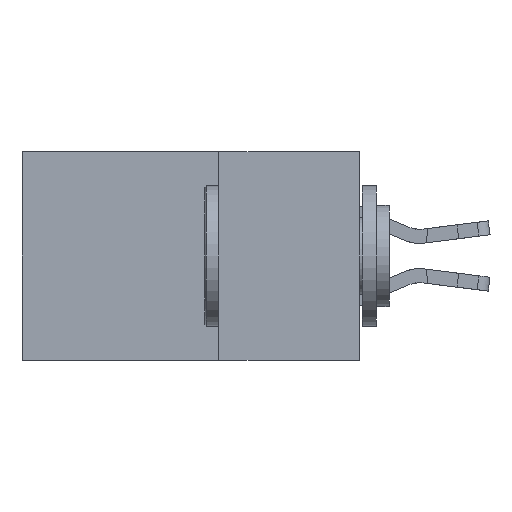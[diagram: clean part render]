
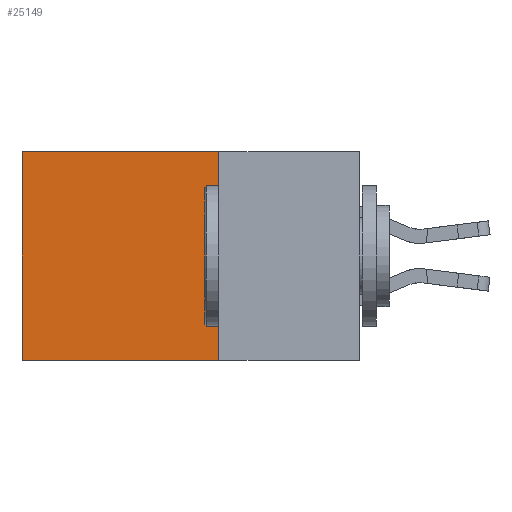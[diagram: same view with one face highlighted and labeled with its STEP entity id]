
A CAD part, left-side view. The second image highlights one B-rep face of the part: STEP entity #25149.
In plain terms, the highlighted planar face has unit normal (-1, 0, 0).
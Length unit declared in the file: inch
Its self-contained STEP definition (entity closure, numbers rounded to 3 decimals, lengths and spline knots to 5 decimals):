
#284 = LINE ( 'NONE', #14519, #10998 ) ;
#887 = FACE_OUTER_BOUND ( 'NONE', #4075, .T. ) ;
#1728 = CARTESIAN_POINT ( 'NONE',  ( 0.2875, 0.25, 0. ) ) ;
#2765 = DIRECTION ( 'NONE',  ( 0., 1., 0. ) ) ;
#3884 = VERTEX_POINT ( 'NONE', #20386 ) ;
#3923 = VERTEX_POINT ( 'NONE', #10736 ) ;
#3927 = EDGE_CURVE ( 'NONE', #3884, #3923, #23245, .T. ) ;
#4075 = EDGE_LOOP ( 'NONE', ( #24114, #11935, #10011, #7638 ) ) ;
#4761 = CARTESIAN_POINT ( 'NONE',  ( 0.2875, 0.25, -0.37 ) ) ;
#4936 = EDGE_CURVE ( 'NONE', #23314, #8956, #9757, .T. ) ;
#5222 = CARTESIAN_POINT ( 'NONE',  ( 0.2875, 0.25, 0. ) ) ;
#5867 = VECTOR ( 'NONE', #2765, 39.37008 ) ;
#6947 = VECTOR ( 'NONE', #14713, 39.37008 ) ;
#7211 = DIRECTION ( 'NONE',  ( 1., 0., 0. ) ) ;
#7638 = ORIENTED_EDGE ( 'NONE', *, *, #24322, .T. ) ;
#8956 = VERTEX_POINT ( 'NONE', #16486 ) ;
#9757 = LINE ( 'NONE', #1728, #19595 ) ;
#10011 = ORIENTED_EDGE ( 'NONE', *, *, #4936, .F. ) ;
#10736 = CARTESIAN_POINT ( 'NONE',  ( 0.2875, 0.6, -0.37 ) ) ;
#10998 = VECTOR ( 'NONE', #16495, 39.37008 ) ;
#11935 = ORIENTED_EDGE ( 'NONE', *, *, #12284, .F. ) ;
#12284 = EDGE_CURVE ( 'NONE', #8956, #3923, #21585, .T. ) ;
#12731 = CARTESIAN_POINT ( 'NONE',  ( 0.2875, 0.6, 0. ) ) ;
#14519 = CARTESIAN_POINT ( 'NONE',  ( 0.2875, 0.25, 0. ) ) ;
#14713 = DIRECTION ( 'NONE',  ( 0., 0., -1. ) ) ;
#15015 = AXIS2_PLACEMENT_3D ( 'NONE', #5222, #7211, #20993 ) ;
#16486 = CARTESIAN_POINT ( 'NONE',  ( 0.2875, 0.25, -0.37 ) ) ;
#16495 = DIRECTION ( 'NONE',  ( 0., 1., 0. ) ) ;
#17162 = PLANE ( 'NONE',  #15015 ) ;
#17691 = DIRECTION ( 'NONE',  ( 0., 0., -1. ) ) ;
#19595 = VECTOR ( 'NONE', #17691, 39.37008 ) ;
#20386 = CARTESIAN_POINT ( 'NONE',  ( 0.2875, 0.6, 0. ) ) ;
#20993 = DIRECTION ( 'NONE',  ( 0., 0., -1. ) ) ;
#21172 = CARTESIAN_POINT ( 'NONE',  ( 0.2875, 0.25, 0. ) ) ;
#21585 = LINE ( 'NONE', #4761, #5867 ) ;
#23245 = LINE ( 'NONE', #12731, #6947 ) ;
#23314 = VERTEX_POINT ( 'NONE', #21172 ) ;
#24114 = ORIENTED_EDGE ( 'NONE', *, *, #3927, .T. ) ;
#24322 = EDGE_CURVE ( 'NONE', #23314, #3884, #284, .T. ) ;
#25149 = ADVANCED_FACE ( 'NONE', ( #887 ), #17162, .F. ) ;
